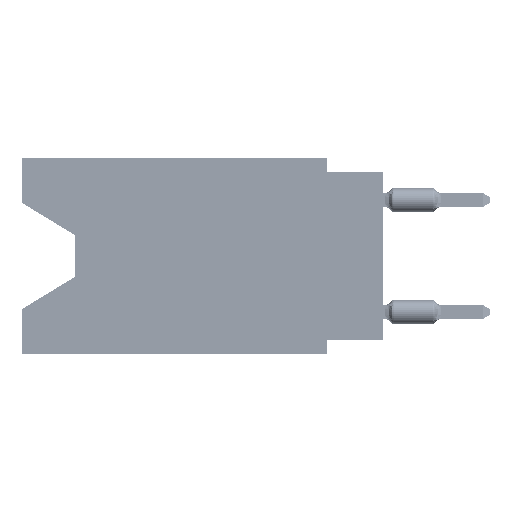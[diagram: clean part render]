
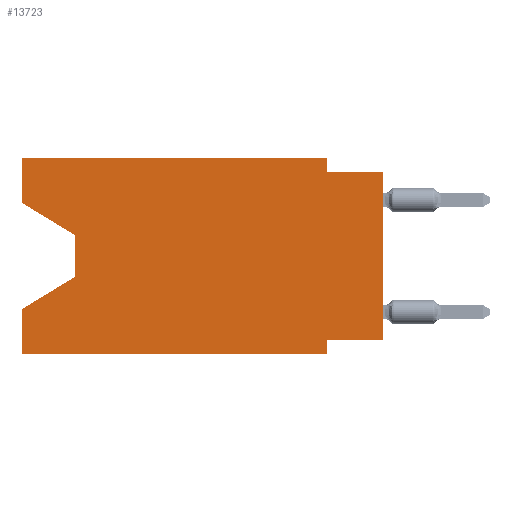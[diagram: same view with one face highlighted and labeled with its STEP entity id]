
A CAD part, left-side view. The second image highlights one B-rep face of the part: STEP entity #13723.
In plain terms, the highlighted planar face has unit normal (-1, 0, 0).
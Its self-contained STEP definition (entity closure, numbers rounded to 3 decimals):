
#2525 = CARTESIAN_POINT ( 'NONE',  ( 0., 16.383, 0. ) ) ;
#2609 = DIRECTION ( 'NONE',  ( 0., 0., -1. ) ) ;
#5346 = CARTESIAN_POINT ( 'NONE',  ( 0., 0., -8.255 ) ) ;
#6518 = EDGE_CURVE ( 'NONE', #85962, #78162, #82872, .T. ) ;
#6882 = CARTESIAN_POINT ( 'NONE',  ( 0., 2.54, 0. ) ) ;
#6906 = ORIENTED_EDGE ( 'NONE', *, *, #17697, .T. ) ;
#7820 = CARTESIAN_POINT ( 'NONE',  ( 0., 2.54, -0.635 ) ) ;
#9512 = CARTESIAN_POINT ( 'NONE',  ( 0., 16.383, -8.89 ) ) ;
#10131 = CARTESIAN_POINT ( 'NONE',  ( 0., 16.383, 0. ) ) ;
#10597 = LINE ( 'NONE', #72763, #104379 ) ;
#11227 = CARTESIAN_POINT ( 'NONE',  ( 0., 16.383, -8.89 ) ) ;
#11255 = VERTEX_POINT ( 'NONE', #109984 ) ;
#13421 = ORIENTED_EDGE ( 'NONE', *, *, #21222, .T. ) ;
#13723 = ADVANCED_FACE ( 'NONE', ( #78856 ), #104055, .F. ) ;
#14574 = AXIS2_PLACEMENT_3D ( 'NONE', #87638, #32515, #51854 ) ;
#15352 = CARTESIAN_POINT ( 'NONE',  ( 0., 13.97, -3.505 ) ) ;
#16099 = DIRECTION ( 'NONE',  ( 0., 0., 1. ) ) ;
#16396 = VERTEX_POINT ( 'NONE', #42954 ) ;
#17697 = EDGE_CURVE ( 'NONE', #62722, #40623, #54059, .T. ) ;
#17714 = CARTESIAN_POINT ( 'NONE',  ( 0., 0., 0. ) ) ;
#18276 = DIRECTION ( 'NONE',  ( 0., 0., 1. ) ) ;
#18594 = EDGE_CURVE ( 'NONE', #25525, #54920, #41769, .T. ) ;
#21222 = EDGE_CURVE ( 'NONE', #11255, #25525, #34871, .T. ) ;
#21642 = EDGE_CURVE ( 'NONE', #26882, #16396, #36448, .T. ) ;
#22503 = VECTOR ( 'NONE', #2609, 1000. ) ;
#23315 = VECTOR ( 'NONE', #81193, 1000. ) ;
#25525 = VERTEX_POINT ( 'NONE', #90119 ) ;
#26882 = VERTEX_POINT ( 'NONE', #88051 ) ;
#30539 = DIRECTION ( 'NONE',  ( 0., -1., 0. ) ) ;
#32515 = DIRECTION ( 'NONE',  ( 1., 0., 0. ) ) ;
#34608 = EDGE_CURVE ( 'NONE', #11255, #85962, #54691, .T. ) ;
#34871 = LINE ( 'NONE', #45410, #23315 ) ;
#36448 = LINE ( 'NONE', #42979, #77658 ) ;
#38284 = DIRECTION ( 'NONE',  ( 0., -1., 0. ) ) ;
#38397 = DIRECTION ( 'NONE',  ( 0., 1., 0. ) ) ;
#38720 = EDGE_CURVE ( 'NONE', #62722, #26882, #40129, .T. ) ;
#38824 = DIRECTION ( 'NONE',  ( 0., 0., 1. ) ) ;
#40030 = ORIENTED_EDGE ( 'NONE', *, *, #21642, .F. ) ;
#40129 = LINE ( 'NONE', #111657, #92558 ) ;
#40380 = ORIENTED_EDGE ( 'NONE', *, *, #93396, .T. ) ;
#40623 = VERTEX_POINT ( 'NONE', #81569 ) ;
#40706 = EDGE_CURVE ( 'NONE', #53685, #40623, #10597, .T. ) ;
#41769 = LINE ( 'NONE', #15352, #86540 ) ;
#42926 = DIRECTION ( 'NONE',  ( 0., 0., -1. ) ) ;
#42954 = CARTESIAN_POINT ( 'NONE',  ( 0., 2.54, -8.89 ) ) ;
#42979 = CARTESIAN_POINT ( 'NONE',  ( 0., 2.54, -8.89 ) ) ;
#45410 = CARTESIAN_POINT ( 'NONE',  ( 0., 16.383, -2.038 ) ) ;
#50818 = CARTESIAN_POINT ( 'NONE',  ( 0., 16.383, -6.852 ) ) ;
#51854 = DIRECTION ( 'NONE',  ( 0., 0., -1. ) ) ;
#53685 = VERTEX_POINT ( 'NONE', #7820 ) ;
#54059 = LINE ( 'NONE', #17714, #75237 ) ;
#54691 = LINE ( 'NONE', #10131, #98014 ) ;
#54920 = VERTEX_POINT ( 'NONE', #115813 ) ;
#57977 = DIRECTION ( 'NONE',  ( 0., 0., -1. ) ) ;
#61131 = ORIENTED_EDGE ( 'NONE', *, *, #38720, .F. ) ;
#62722 = VERTEX_POINT ( 'NONE', #5346 ) ;
#63785 = CARTESIAN_POINT ( 'NONE',  ( 0., 16.383, 0. ) ) ;
#65924 = LINE ( 'NONE', #72396, #22503 ) ;
#69355 = VERTEX_POINT ( 'NONE', #9512 ) ;
#71723 = LINE ( 'NONE', #107470, #98276 ) ;
#71992 = ORIENTED_EDGE ( 'NONE', *, *, #82960, .F. ) ;
#72396 = CARTESIAN_POINT ( 'NONE',  ( 0., 2.54, 0. ) ) ;
#72763 = CARTESIAN_POINT ( 'NONE',  ( 0., 0., -0.635 ) ) ;
#75237 = VECTOR ( 'NONE', #18276, 1000. ) ;
#77658 = VECTOR ( 'NONE', #57977, 1000. ) ;
#78162 = VERTEX_POINT ( 'NONE', #6882 ) ;
#78856 = FACE_OUTER_BOUND ( 'NONE', #108567, .T. ) ;
#80494 = ORIENTED_EDGE ( 'NONE', *, *, #106870, .F. ) ;
#81193 = DIRECTION ( 'NONE',  ( 0., -0.855, -0.519 ) ) ;
#81569 = CARTESIAN_POINT ( 'NONE',  ( 0., 0., -0.635 ) ) ;
#82182 = VECTOR ( 'NONE', #16099, 1000. ) ;
#82449 = ORIENTED_EDGE ( 'NONE', *, *, #6518, .F. ) ;
#82872 = LINE ( 'NONE', #2525, #106092 ) ;
#82960 = EDGE_CURVE ( 'NONE', #69355, #86370, #86494, .T. ) ;
#83617 = EDGE_CURVE ( 'NONE', #69355, #16396, #110277, .T. ) ;
#84193 = VECTOR ( 'NONE', #30539, 1000. ) ;
#85891 = ORIENTED_EDGE ( 'NONE', *, *, #34608, .F. ) ;
#85962 = VERTEX_POINT ( 'NONE', #63785 ) ;
#86370 = VERTEX_POINT ( 'NONE', #50818 ) ;
#86484 = ORIENTED_EDGE ( 'NONE', *, *, #40706, .F. ) ;
#86494 = LINE ( 'NONE', #105240, #82182 ) ;
#86540 = VECTOR ( 'NONE', #42926, 1000. ) ;
#87638 = CARTESIAN_POINT ( 'NONE',  ( 0., 16.383, 0. ) ) ;
#88051 = CARTESIAN_POINT ( 'NONE',  ( 0., 2.54, -8.255 ) ) ;
#89895 = DIRECTION ( 'NONE',  ( 0., 0.855, -0.519 ) ) ;
#90119 = CARTESIAN_POINT ( 'NONE',  ( 0., 13.97, -3.505 ) ) ;
#92558 = VECTOR ( 'NONE', #38397, 1000. ) ;
#93396 = EDGE_CURVE ( 'NONE', #54920, #86370, #71723, .T. ) ;
#98014 = VECTOR ( 'NONE', #38824, 1000. ) ;
#98276 = VECTOR ( 'NONE', #89895, 1000. ) ;
#98735 = ORIENTED_EDGE ( 'NONE', *, *, #18594, .T. ) ;
#104055 = PLANE ( 'NONE',  #14574 ) ;
#104379 = VECTOR ( 'NONE', #108517, 1000. ) ;
#105240 = CARTESIAN_POINT ( 'NONE',  ( 0., 16.383, 0. ) ) ;
#106092 = VECTOR ( 'NONE', #38284, 1000. ) ;
#106870 = EDGE_CURVE ( 'NONE', #78162, #53685, #65924, .T. ) ;
#107470 = CARTESIAN_POINT ( 'NONE',  ( 0., 13.97, -5.385 ) ) ;
#108517 = DIRECTION ( 'NONE',  ( 0., -1., 0. ) ) ;
#108567 = EDGE_LOOP ( 'NONE', ( #13421, #98735, #40380, #71992, #110862, #40030, #61131, #6906, #86484, #80494, #82449, #85891 ) ) ;
#109984 = CARTESIAN_POINT ( 'NONE',  ( 0., 16.383, -2.038 ) ) ;
#110277 = LINE ( 'NONE', #11227, #84193 ) ;
#110862 = ORIENTED_EDGE ( 'NONE', *, *, #83617, .T. ) ;
#111657 = CARTESIAN_POINT ( 'NONE',  ( 0., 0., -8.255 ) ) ;
#115813 = CARTESIAN_POINT ( 'NONE',  ( 0., 13.97, -5.385 ) ) ;
